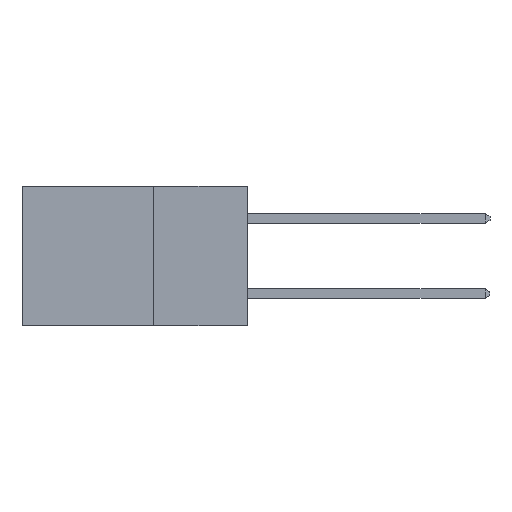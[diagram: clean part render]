
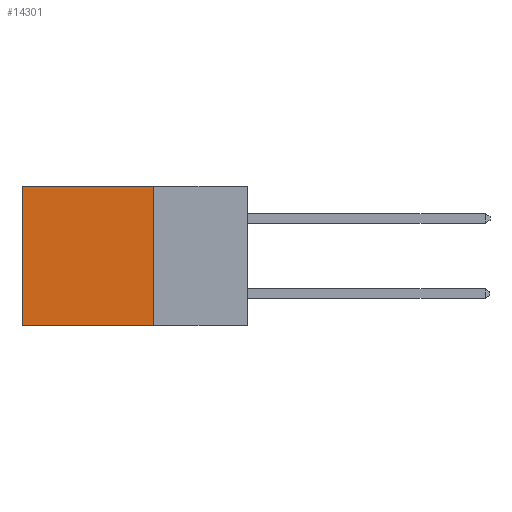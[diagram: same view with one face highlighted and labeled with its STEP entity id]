
A CAD part, left-side view. The second image highlights one B-rep face of the part: STEP entity #14301.
In plain terms, the highlighted planar face has unit normal (-1, 0, 0).
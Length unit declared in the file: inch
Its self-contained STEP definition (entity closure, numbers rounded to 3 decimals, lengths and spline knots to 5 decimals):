
#3266 = DIRECTION ( 'NONE',  ( 0., 0., -1. ) ) ;
#4211 = ORIENTED_EDGE ( 'NONE', *, *, #22423, .F. ) ;
#4358 = VECTOR ( 'NONE', #3266, 39.37008 ) ;
#4444 = VERTEX_POINT ( 'NONE', #21658 ) ;
#6262 = VECTOR ( 'NONE', #27854, 39.37008 ) ;
#6817 = FACE_OUTER_BOUND ( 'NONE', #13116, .T. ) ;
#7322 = VERTEX_POINT ( 'NONE', #15207 ) ;
#8291 = CARTESIAN_POINT ( 'NONE',  ( 0.298, 0.6, 0. ) ) ;
#8618 = CARTESIAN_POINT ( 'NONE',  ( 0.298, 0.25, -0.37 ) ) ;
#13061 = DIRECTION ( 'NONE',  ( 0., 0., -1. ) ) ;
#13116 = EDGE_LOOP ( 'NONE', ( #24508, #4211, #27948, #19453 ) ) ;
#13577 = LINE ( 'NONE', #8618, #6262 ) ;
#14301 = ADVANCED_FACE ( 'NONE', ( #6817 ), #25052, .F. ) ;
#15207 = CARTESIAN_POINT ( 'NONE',  ( 0.298, 0.6, -0.37 ) ) ;
#16136 = EDGE_CURVE ( 'NONE', #4444, #24256, #30015, .T. ) ;
#16714 = DIRECTION ( 'NONE',  ( 0., 1., 0. ) ) ;
#18276 = LINE ( 'NONE', #18772, #19037 ) ;
#18772 = CARTESIAN_POINT ( 'NONE',  ( 0.298, 0.6, 0. ) ) ;
#19037 = VECTOR ( 'NONE', #30593, 39.37008 ) ;
#19453 = ORIENTED_EDGE ( 'NONE', *, *, #20094, .T. ) ;
#20094 = EDGE_CURVE ( 'NONE', #4444, #22341, #29006, .T. ) ;
#20124 = CARTESIAN_POINT ( 'NONE',  ( 0.298, 0.25, 0. ) ) ;
#21658 = CARTESIAN_POINT ( 'NONE',  ( 0.298, 0.25, 0. ) ) ;
#22341 = VERTEX_POINT ( 'NONE', #8291 ) ;
#22423 = EDGE_CURVE ( 'NONE', #24256, #7322, #13577, .T. ) ;
#22788 = CARTESIAN_POINT ( 'NONE',  ( 0.298, 0.25, 0. ) ) ;
#22935 = AXIS2_PLACEMENT_3D ( 'NONE', #20124, #27383, #13061 ) ;
#23870 = CARTESIAN_POINT ( 'NONE',  ( 0.298, 0.25, 0. ) ) ;
#24256 = VERTEX_POINT ( 'NONE', #29912 ) ;
#24508 = ORIENTED_EDGE ( 'NONE', *, *, #29310, .T. ) ;
#25052 = PLANE ( 'NONE',  #22935 ) ;
#27383 = DIRECTION ( 'NONE',  ( 1., 0., 0. ) ) ;
#27854 = DIRECTION ( 'NONE',  ( 0., 1., 0. ) ) ;
#27948 = ORIENTED_EDGE ( 'NONE', *, *, #16136, .F. ) ;
#28263 = VECTOR ( 'NONE', #16714, 39.37008 ) ;
#29006 = LINE ( 'NONE', #23870, #28263 ) ;
#29310 = EDGE_CURVE ( 'NONE', #22341, #7322, #18276, .T. ) ;
#29912 = CARTESIAN_POINT ( 'NONE',  ( 0.298, 0.25, -0.37 ) ) ;
#30015 = LINE ( 'NONE', #22788, #4358 ) ;
#30593 = DIRECTION ( 'NONE',  ( 0., 0., -1. ) ) ;
